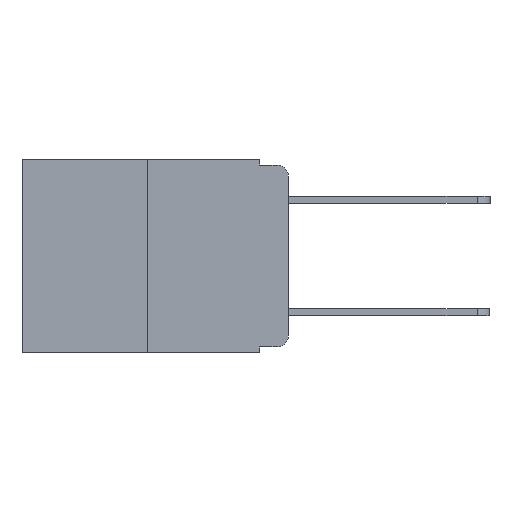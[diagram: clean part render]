
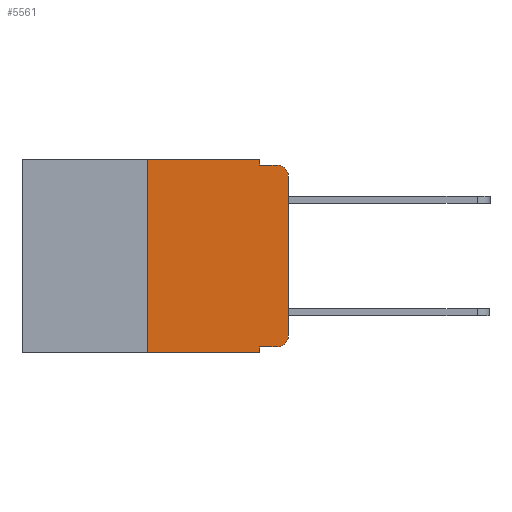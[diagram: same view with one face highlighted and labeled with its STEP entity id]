
A CAD part, left-side view. The second image highlights one B-rep face of the part: STEP entity #5561.
In plain terms, the highlighted planar face has unit normal (-1, 0, 0).
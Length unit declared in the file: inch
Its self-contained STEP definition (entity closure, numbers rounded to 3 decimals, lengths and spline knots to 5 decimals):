
#3 = VECTOR ( 'NONE', #10525, 39.37008 ) ;
#82 = AXIS2_PLACEMENT_3D ( 'NONE', #22031, #11584, #970 ) ;
#466 = EDGE_CURVE ( 'NONE', #1138, #3939, #19137, .T. ) ;
#865 = LINE ( 'NONE', #20173, #5033 ) ;
#872 = DIRECTION ( 'NONE',  ( 0., 0., -1. ) ) ;
#970 = DIRECTION ( 'NONE',  ( 0., 0., -1. ) ) ;
#1040 = EDGE_CURVE ( 'NONE', #10275, #12342, #17238, .T. ) ;
#1046 = CARTESIAN_POINT ( 'NONE',  ( 0., 0.051, 0. ) ) ;
#1138 = VERTEX_POINT ( 'NONE', #2383 ) ;
#1644 = CIRCLE ( 'NONE', #5751, 0.02 ) ;
#1924 = FACE_OUTER_BOUND ( 'NONE', #17635, .T. ) ;
#2152 = VECTOR ( 'NONE', #6448, 39.37008 ) ;
#2383 = CARTESIAN_POINT ( 'NONE',  ( 0., 0.25, 0. ) ) ;
#2543 = DIRECTION ( 'NONE',  ( 0., 0., 1. ) ) ;
#3497 = CIRCLE ( 'NONE', #82, 0.02 ) ;
#3939 = VERTEX_POINT ( 'NONE', #8391 ) ;
#5033 = VECTOR ( 'NONE', #11488, 39.37008 ) ;
#5132 = VECTOR ( 'NONE', #17749, 39.37008 ) ;
#5184 = LINE ( 'NONE', #17114, #18638 ) ;
#5561 = ADVANCED_FACE ( 'NONE', ( #1924 ), #17617, .F. ) ;
#5582 = VERTEX_POINT ( 'NONE', #17691 ) ;
#5751 = AXIS2_PLACEMENT_3D ( 'NONE', #21932, #11492, #872 ) ;
#6448 = DIRECTION ( 'NONE',  ( 0., 0., -1. ) ) ;
#7406 = EDGE_CURVE ( 'NONE', #11911, #5582, #5184, .T. ) ;
#7455 = ORIENTED_EDGE ( 'NONE', *, *, #21362, .F. ) ;
#7765 = VERTEX_POINT ( 'NONE', #16259 ) ;
#8266 = ORIENTED_EDGE ( 'NONE', *, *, #19077, .F. ) ;
#8391 = CARTESIAN_POINT ( 'NONE',  ( 0., 0.051, 0. ) ) ;
#8529 = EDGE_CURVE ( 'NONE', #11911, #1138, #10688, .T. ) ;
#8911 = DIRECTION ( 'NONE',  ( 0., 0., -1. ) ) ;
#8973 = CARTESIAN_POINT ( 'NONE',  ( 0., 0., -0.313 ) ) ;
#9177 = LINE ( 'NONE', #1046, #17906 ) ;
#9573 = CARTESIAN_POINT ( 'NONE',  ( 0., 0.25, 0. ) ) ;
#9665 = CARTESIAN_POINT ( 'NONE',  ( 0., 0., 0. ) ) ;
#10205 = CARTESIAN_POINT ( 'NONE',  ( 0., 0.25, -0.343 ) ) ;
#10275 = VERTEX_POINT ( 'NONE', #8973 ) ;
#10525 = DIRECTION ( 'NONE',  ( 0., -1., 0. ) ) ;
#10536 = EDGE_CURVE ( 'NONE', #12122, #21629, #865, .T. ) ;
#10610 = CARTESIAN_POINT ( 'NONE',  ( 0., 0.473, 0. ) ) ;
#10688 = LINE ( 'NONE', #9573, #14779 ) ;
#11412 = ORIENTED_EDGE ( 'NONE', *, *, #7406, .T. ) ;
#11488 = DIRECTION ( 'NONE',  ( 0., -1., 0. ) ) ;
#11492 = DIRECTION ( 'NONE',  ( -1., 0., 0. ) ) ;
#11553 = LINE ( 'NONE', #17065, #2152 ) ;
#11584 = DIRECTION ( 'NONE',  ( -1., 0., 0. ) ) ;
#11790 = EDGE_CURVE ( 'NONE', #3939, #7765, #9177, .T. ) ;
#11911 = VERTEX_POINT ( 'NONE', #10205 ) ;
#12122 = VERTEX_POINT ( 'NONE', #19438 ) ;
#12280 = CARTESIAN_POINT ( 'NONE',  ( 0., 0.051, -0.01 ) ) ;
#12328 = EDGE_CURVE ( 'NONE', #21629, #10275, #1644, .T. ) ;
#12342 = VERTEX_POINT ( 'NONE', #14927 ) ;
#12463 = CARTESIAN_POINT ( 'NONE',  ( 0., 0.473, 0. ) ) ;
#14034 = ORIENTED_EDGE ( 'NONE', *, *, #11790, .F. ) ;
#14146 = ORIENTED_EDGE ( 'NONE', *, *, #8529, .F. ) ;
#14241 = EDGE_CURVE ( 'NONE', #12342, #15104, #3497, .T. ) ;
#14779 = VECTOR ( 'NONE', #2543, 39.37008 ) ;
#14927 = CARTESIAN_POINT ( 'NONE',  ( 0., 0., -0.03 ) ) ;
#15104 = VERTEX_POINT ( 'NONE', #17490 ) ;
#15563 = ORIENTED_EDGE ( 'NONE', *, *, #466, .F. ) ;
#16259 = CARTESIAN_POINT ( 'NONE',  ( 0., 0.051, -0.01 ) ) ;
#16689 = VECTOR ( 'NONE', #20377, 39.37008 ) ;
#17065 = CARTESIAN_POINT ( 'NONE',  ( 0., 0.051, 0. ) ) ;
#17114 = CARTESIAN_POINT ( 'NONE',  ( 0., 0.473, -0.343 ) ) ;
#17238 = LINE ( 'NONE', #9665, #16689 ) ;
#17490 = CARTESIAN_POINT ( 'NONE',  ( 0., 0.02, -0.01 ) ) ;
#17596 = AXIS2_PLACEMENT_3D ( 'NONE', #10610, #19372, #8911 ) ;
#17617 = PLANE ( 'NONE',  #17596 ) ;
#17635 = EDGE_LOOP ( 'NONE', ( #21677, #19267, #8266, #14034, #15563, #14146, #11412, #7455, #21768, #17804 ) ) ;
#17691 = CARTESIAN_POINT ( 'NONE',  ( 0., 0.051, -0.343 ) ) ;
#17749 = DIRECTION ( 'NONE',  ( 0., -1., 0. ) ) ;
#17804 = ORIENTED_EDGE ( 'NONE', *, *, #12328, .T. ) ;
#17906 = VECTOR ( 'NONE', #22106, 39.37008 ) ;
#18186 = LINE ( 'NONE', #12280, #3 ) ;
#18638 = VECTOR ( 'NONE', #18860, 39.37008 ) ;
#18860 = DIRECTION ( 'NONE',  ( 0., -1., 0. ) ) ;
#19077 = EDGE_CURVE ( 'NONE', #7765, #15104, #18186, .T. ) ;
#19137 = LINE ( 'NONE', #12463, #5132 ) ;
#19267 = ORIENTED_EDGE ( 'NONE', *, *, #14241, .T. ) ;
#19372 = DIRECTION ( 'NONE',  ( 1., 0., 0. ) ) ;
#19438 = CARTESIAN_POINT ( 'NONE',  ( 0., 0.051, -0.333 ) ) ;
#19573 = CARTESIAN_POINT ( 'NONE',  ( 0., 0.02, -0.333 ) ) ;
#20173 = CARTESIAN_POINT ( 'NONE',  ( 0., 0.051, -0.333 ) ) ;
#20377 = DIRECTION ( 'NONE',  ( 0., 0., 1. ) ) ;
#21362 = EDGE_CURVE ( 'NONE', #12122, #5582, #11553, .T. ) ;
#21629 = VERTEX_POINT ( 'NONE', #19573 ) ;
#21677 = ORIENTED_EDGE ( 'NONE', *, *, #1040, .T. ) ;
#21768 = ORIENTED_EDGE ( 'NONE', *, *, #10536, .T. ) ;
#21932 = CARTESIAN_POINT ( 'NONE',  ( 0., 0.02, -0.313 ) ) ;
#22031 = CARTESIAN_POINT ( 'NONE',  ( 0., 0.02, -0.03 ) ) ;
#22106 = DIRECTION ( 'NONE',  ( 0., 0., -1. ) ) ;
